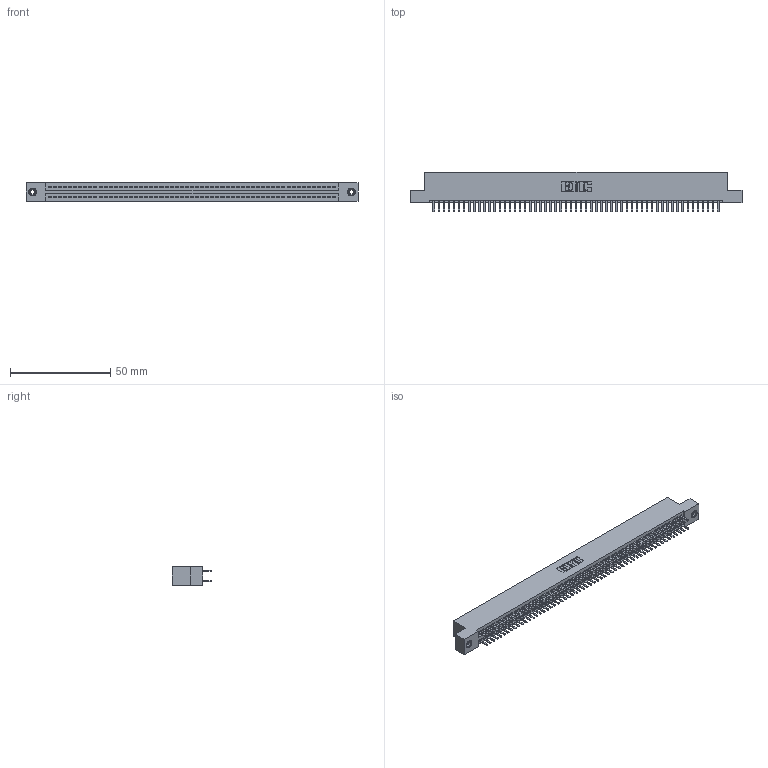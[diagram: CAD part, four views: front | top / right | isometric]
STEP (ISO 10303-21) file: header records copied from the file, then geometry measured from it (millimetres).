
FILE_DESCRIPTION (( 'STEP AP203' ), '1' );
FILE_NAME ('395-114-520-208.STEP', '2019-10-27T16:55:46', ( '' ), ( '' ), 'SwSTEP 2.0', 'SolidWorks 2016', '' );
FILE_SCHEMA (( 'CONFIG_CONTROL_DESIGN' ));
Length unit declared in the file: inch
Products named in the file (4): 345 Part_Flush Mounting Lugs - 0.156 Dia-TI; 345-292-001_345-293-120; 345-250-001_345-250-003-102; 395-114-520-208
Assembly tree (117 placements, depth 2):
  395-114-520-208
    345 Part_Flush Mounting Lugs - 0.156 Dia-TI
    345-292-001_345-293-120  x114
    345-250-001_345-250-003-102  x2
Bounding box: 165.99 x 19.68 x 9.4 mm (x, y, z)
Volume: 16206.9 mm3; surface area: 24153.9 mm2
Topology: 117 solids, 117 shells, 6342 faces, 18375 edges, 11938 vertices
Faces by surface type: plane 4102, cylinder 2224, cone 12, torus 4
Entity records: 44004 total; most frequent: CARTESIAN_POINT 7355, ORIENTED_EDGE 7270, DIRECTION 6481, EDGE_CURVE 3635, LINE 3251, VECTOR 3251, VERTEX_POINT 2416, AXIS2_PLACEMENT_3D 1615
